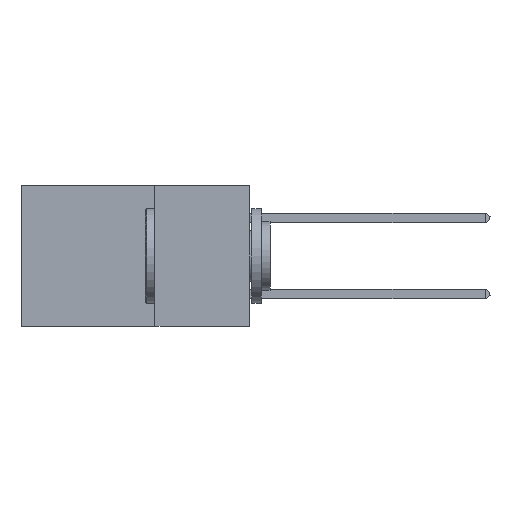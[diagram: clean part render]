
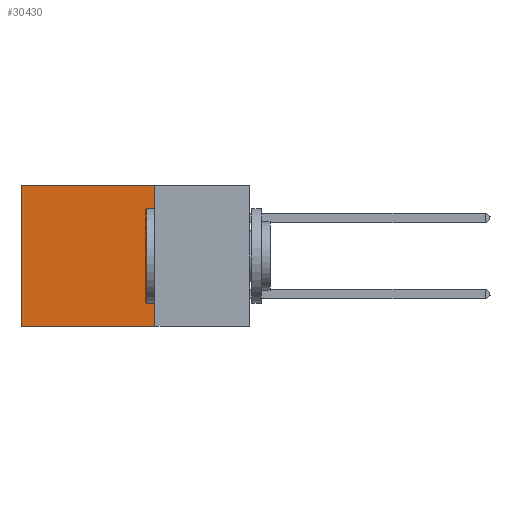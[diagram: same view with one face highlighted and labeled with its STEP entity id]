
A CAD part, left-side view. The second image highlights one B-rep face of the part: STEP entity #30430.
In plain terms, the highlighted planar face has unit normal (-1, 0, 0).
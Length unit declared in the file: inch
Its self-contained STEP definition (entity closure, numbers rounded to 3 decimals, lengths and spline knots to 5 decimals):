
#3127 = VERTEX_POINT ( 'NONE', #36854 ) ;
#3660 = VERTEX_POINT ( 'NONE', #12386 ) ;
#5085 = ORIENTED_EDGE ( 'NONE', *, *, #11984, .F. ) ;
#5663 = LINE ( 'NONE', #34803, #27278 ) ;
#6678 = VECTOR ( 'NONE', #25255, 39.37008 ) ;
#7870 = ORIENTED_EDGE ( 'NONE', *, *, #24591, .T. ) ;
#9167 = LINE ( 'NONE', #34153, #37325 ) ;
#11984 = EDGE_CURVE ( 'NONE', #13902, #19060, #5663, .T. ) ;
#12386 = CARTESIAN_POINT ( 'NONE',  ( 0.2875, 0.6, 0. ) ) ;
#13285 = CARTESIAN_POINT ( 'NONE',  ( 0.2875, 0.6, 0. ) ) ;
#13902 = VERTEX_POINT ( 'NONE', #37166 ) ;
#14503 = ORIENTED_EDGE ( 'NONE', *, *, #20703, .F. ) ;
#15465 = CARTESIAN_POINT ( 'NONE',  ( 0.2875, 0.25, 0. ) ) ;
#16542 = CARTESIAN_POINT ( 'NONE',  ( 0.2875, 0.6, -0.37 ) ) ;
#18608 = PLANE ( 'NONE',  #23716 ) ;
#19060 = VERTEX_POINT ( 'NONE', #16542 ) ;
#20703 = EDGE_CURVE ( 'NONE', #3127, #13902, #30105, .T. ) ;
#20724 = EDGE_LOOP ( 'NONE', ( #7870, #5085, #14503, #33799 ) ) ;
#20764 = CARTESIAN_POINT ( 'NONE',  ( 0.2875, 0.25, 0. ) ) ;
#22137 = VECTOR ( 'NONE', #35686, 39.37008 ) ;
#22670 = LINE ( 'NONE', #13285, #6678 ) ;
#23716 = AXIS2_PLACEMENT_3D ( 'NONE', #15465, #30552, #36548 ) ;
#24591 = EDGE_CURVE ( 'NONE', #3660, #19060, #22670, .T. ) ;
#25255 = DIRECTION ( 'NONE',  ( 0., 0., -1. ) ) ;
#27278 = VECTOR ( 'NONE', #28507, 39.37008 ) ;
#28501 = DIRECTION ( 'NONE',  ( 0., 1., 0. ) ) ;
#28507 = DIRECTION ( 'NONE',  ( 0., 1., 0. ) ) ;
#30105 = LINE ( 'NONE', #20764, #22137 ) ;
#30430 = ADVANCED_FACE ( 'NONE', ( #31395 ), #18608, .F. ) ;
#30552 = DIRECTION ( 'NONE',  ( 1., 0., 0. ) ) ;
#31395 = FACE_OUTER_BOUND ( 'NONE', #20724, .T. ) ;
#32613 = EDGE_CURVE ( 'NONE', #3127, #3660, #9167, .T. ) ;
#33799 = ORIENTED_EDGE ( 'NONE', *, *, #32613, .T. ) ;
#34153 = CARTESIAN_POINT ( 'NONE',  ( 0.2875, 0.25, 0. ) ) ;
#34803 = CARTESIAN_POINT ( 'NONE',  ( 0.2875, 0.25, -0.37 ) ) ;
#35686 = DIRECTION ( 'NONE',  ( 0., 0., -1. ) ) ;
#36548 = DIRECTION ( 'NONE',  ( 0., 0., -1. ) ) ;
#36854 = CARTESIAN_POINT ( 'NONE',  ( 0.2875, 0.25, 0. ) ) ;
#37166 = CARTESIAN_POINT ( 'NONE',  ( 0.2875, 0.25, -0.37 ) ) ;
#37325 = VECTOR ( 'NONE', #28501, 39.37008 ) ;
